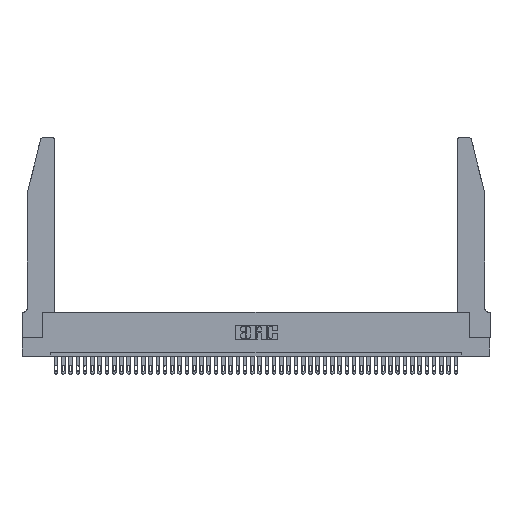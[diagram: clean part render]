
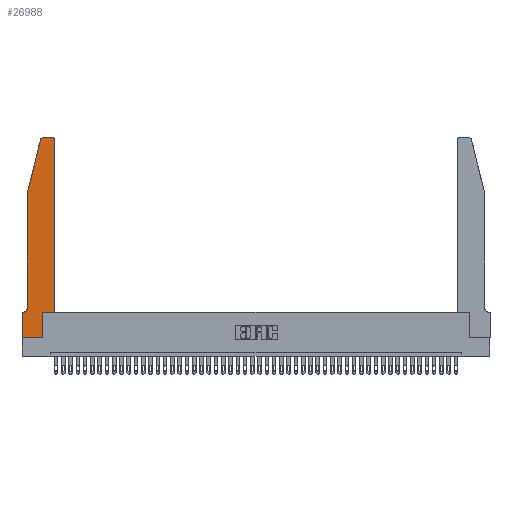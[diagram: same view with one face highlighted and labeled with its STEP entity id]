
A CAD part, top view. The second image highlights one B-rep face of the part: STEP entity #26988.
In plain terms, the highlighted planar face has unit normal (0, 0, 1).
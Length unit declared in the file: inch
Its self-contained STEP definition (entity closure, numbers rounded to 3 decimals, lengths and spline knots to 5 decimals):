
#371 = VERTEX_POINT ( 'NONE', #32483 ) ;
#592 = EDGE_CURVE ( 'NONE', #25665, #30814, #17635, .T. ) ;
#1153 = VERTEX_POINT ( 'NONE', #32497 ) ;
#1251 = CARTESIAN_POINT ( 'NONE',  ( 0.4505, 2.72, 0.37 ) ) ;
#1559 = EDGE_CURVE ( 'NONE', #17417, #25665, #8366, .T. ) ;
#1777 = CARTESIAN_POINT ( 'NONE',  ( 0., 0., 0.37 ) ) ;
#2017 = DIRECTION ( 'NONE',  ( 0., 1., 0. ) ) ;
#2278 = ORIENTED_EDGE ( 'NONE', *, *, #44616, .T. ) ;
#2414 = DIRECTION ( 'NONE',  ( 1., 0., 0. ) ) ;
#2507 = VECTOR ( 'NONE', #15061, 39.37008 ) ;
#2694 = DIRECTION ( 'NONE',  ( 1., 0., 0. ) ) ;
#3032 = DIRECTION ( 'NONE',  ( 0., 0., 1. ) ) ;
#3326 = VERTEX_POINT ( 'NONE', #14627 ) ;
#3653 = AXIS2_PLACEMENT_3D ( 'NONE', #43778, #43934, #2694 ) ;
#4521 = EDGE_CURVE ( 'NONE', #10692, #19245, #15710, .T. ) ;
#5145 = CARTESIAN_POINT ( 'NONE',  ( 0.4505, 0.35, 0.37 ) ) ;
#5306 = VECTOR ( 'NONE', #17128, 39.37008 ) ;
#5864 = CARTESIAN_POINT ( 'NONE',  ( 0.4505, 0.35, 0.37 ) ) ;
#6525 = CARTESIAN_POINT ( 'NONE',  ( 0.0055, 0.35, 0.37 ) ) ;
#7644 = EDGE_CURVE ( 'NONE', #11097, #10396, #30692, .T. ) ;
#8121 = AXIS2_PLACEMENT_3D ( 'NONE', #9512, #3032, #2414 ) ;
#8366 = CIRCLE ( 'NONE', #23593, 0.03 ) ;
#8629 = CARTESIAN_POINT ( 'NONE',  ( 0.284, 2.72, 0.37 ) ) ;
#9006 = EDGE_CURVE ( 'NONE', #23470, #18108, #40958, .T. ) ;
#9471 = VECTOR ( 'NONE', #35552, 39.37008 ) ;
#9512 = CARTESIAN_POINT ( 'NONE',  ( 0., 0.35, 0.37 ) ) ;
#9662 = ORIENTED_EDGE ( 'NONE', *, *, #21331, .T. ) ;
#9673 = PLANE ( 'NONE',  #8121 ) ;
#9804 = DIRECTION ( 'NONE',  ( 1., 0., 0. ) ) ;
#10240 = ORIENTED_EDGE ( 'NONE', *, *, #33646, .T. ) ;
#10396 = VERTEX_POINT ( 'NONE', #38653 ) ;
#10514 = AXIS2_PLACEMENT_3D ( 'NONE', #27894, #14311, #34888 ) ;
#10692 = VERTEX_POINT ( 'NONE', #6525 ) ;
#11011 = LINE ( 'NONE', #29837, #9471 ) ;
#11097 = VERTEX_POINT ( 'NONE', #1777 ) ;
#12189 = ORIENTED_EDGE ( 'NONE', *, *, #9006, .T. ) ;
#13557 = LINE ( 'NONE', #32917, #22737 ) ;
#13656 = VECTOR ( 'NONE', #32850, 39.37008 ) ;
#14247 = ORIENTED_EDGE ( 'NONE', *, *, #39516, .T. ) ;
#14259 = CIRCLE ( 'NONE', #10514, 0.07 ) ;
#14311 = DIRECTION ( 'NONE',  ( 0., 0., -1. ) ) ;
#14452 = CARTESIAN_POINT ( 'NONE',  ( 0.0755, 0.35, 0.37 ) ) ;
#14588 = CARTESIAN_POINT ( 'NONE',  ( 0.25487, 2.72718, 0.37 ) ) ;
#14627 = CARTESIAN_POINT ( 'NONE',  ( 0.4205, 2.75, 0.37 ) ) ;
#14657 = LINE ( 'NONE', #43055, #13656 ) ;
#15061 = DIRECTION ( 'NONE',  ( 1., 0., 0. ) ) ;
#15710 = LINE ( 'NONE', #14452, #38529 ) ;
#16889 = CARTESIAN_POINT ( 'NONE',  ( 0.284, 2.75, 0.37 ) ) ;
#17128 = DIRECTION ( 'NONE',  ( -1., 0., 0. ) ) ;
#17417 = VERTEX_POINT ( 'NONE', #16889 ) ;
#17635 = LINE ( 'NONE', #34402, #20882 ) ;
#18108 = VERTEX_POINT ( 'NONE', #1251 ) ;
#19245 = VERTEX_POINT ( 'NONE', #19876 ) ;
#19876 = CARTESIAN_POINT ( 'NONE',  ( 0., 0.35, 0.37 ) ) ;
#20882 = VECTOR ( 'NONE', #24058, 39.37008 ) ;
#21206 = VECTOR ( 'NONE', #9804, 39.37008 ) ;
#21331 = EDGE_CURVE ( 'NONE', #3326, #17417, #41724, .T. ) ;
#21405 = CARTESIAN_POINT ( 'NONE',  ( 0.0755, 2., 0.37 ) ) ;
#21649 = CIRCLE ( 'NONE', #3653, 0.03 ) ;
#22273 = ORIENTED_EDGE ( 'NONE', *, *, #4521, .T. ) ;
#22362 = VECTOR ( 'NONE', #41183, 39.37008 ) ;
#22737 = VECTOR ( 'NONE', #2017, 39.37008 ) ;
#23470 = VERTEX_POINT ( 'NONE', #5145 ) ;
#23593 = AXIS2_PLACEMENT_3D ( 'NONE', #8629, #32245, #25741 ) ;
#23840 = CARTESIAN_POINT ( 'NONE',  ( 0.4505, 0.35, 0.37 ) ) ;
#24058 = DIRECTION ( 'NONE',  ( -0.239, -0.971, 0. ) ) ;
#24109 = EDGE_CURVE ( 'NONE', #30814, #1153, #11011, .T. ) ;
#24546 = LINE ( 'NONE', #5864, #21206 ) ;
#25665 = VERTEX_POINT ( 'NONE', #14588 ) ;
#25741 = DIRECTION ( 'NONE',  ( 1., 0., 0. ) ) ;
#26988 = ADVANCED_FACE ( 'NONE', ( #29874 ), #9673, .T. ) ;
#27508 = CARTESIAN_POINT ( 'NONE',  ( 0.2605, 2.75, 0.37 ) ) ;
#27894 = CARTESIAN_POINT ( 'NONE',  ( 0.0055, 0.42, 0.37 ) ) ;
#29837 = CARTESIAN_POINT ( 'NONE',  ( 0.0755, 2., 0.37 ) ) ;
#29874 = FACE_OUTER_BOUND ( 'NONE', #32656, .T. ) ;
#30692 = LINE ( 'NONE', #44922, #2507 ) ;
#30759 = ORIENTED_EDGE ( 'NONE', *, *, #1559, .T. ) ;
#30814 = VERTEX_POINT ( 'NONE', #21405 ) ;
#32245 = DIRECTION ( 'NONE',  ( 0., 0., 1. ) ) ;
#32483 = CARTESIAN_POINT ( 'NONE',  ( 0.2865, 0.35, 0.37 ) ) ;
#32497 = CARTESIAN_POINT ( 'NONE',  ( 0.0755, 0.42, 0.37 ) ) ;
#32656 = EDGE_LOOP ( 'NONE', ( #9662, #30759, #41890, #44397, #39322, #22273, #2278, #43233, #14247, #10240, #12189, #44959 ) ) ;
#32797 = EDGE_CURVE ( 'NONE', #1153, #10692, #14259, .T. ) ;
#32850 = DIRECTION ( 'NONE',  ( 0., -1., 0. ) ) ;
#32917 = CARTESIAN_POINT ( 'NONE',  ( 0.2865, 0.35, 0.37 ) ) ;
#33646 = EDGE_CURVE ( 'NONE', #371, #23470, #24546, .T. ) ;
#34402 = CARTESIAN_POINT ( 'NONE',  ( 0.0755, 2., 0.37 ) ) ;
#34888 = DIRECTION ( 'NONE',  ( -1., 0., 0. ) ) ;
#35039 = EDGE_CURVE ( 'NONE', #18108, #3326, #21649, .T. ) ;
#35552 = DIRECTION ( 'NONE',  ( 0., -1., 0. ) ) ;
#38529 = VECTOR ( 'NONE', #38939, 39.37008 ) ;
#38653 = CARTESIAN_POINT ( 'NONE',  ( 0.2865, 0., 0.37 ) ) ;
#38939 = DIRECTION ( 'NONE',  ( -1., 0., 0. ) ) ;
#39322 = ORIENTED_EDGE ( 'NONE', *, *, #32797, .T. ) ;
#39516 = EDGE_CURVE ( 'NONE', #10396, #371, #13557, .T. ) ;
#40958 = LINE ( 'NONE', #23840, #22362 ) ;
#41183 = DIRECTION ( 'NONE',  ( 0., 1., 0. ) ) ;
#41724 = LINE ( 'NONE', #27508, #5306 ) ;
#41890 = ORIENTED_EDGE ( 'NONE', *, *, #592, .T. ) ;
#43055 = CARTESIAN_POINT ( 'NONE',  ( 0., 0., 0.37 ) ) ;
#43233 = ORIENTED_EDGE ( 'NONE', *, *, #7644, .T. ) ;
#43778 = CARTESIAN_POINT ( 'NONE',  ( 0.4205, 2.72, 0.37 ) ) ;
#43934 = DIRECTION ( 'NONE',  ( 0., 0., 1. ) ) ;
#44397 = ORIENTED_EDGE ( 'NONE', *, *, #24109, .T. ) ;
#44616 = EDGE_CURVE ( 'NONE', #19245, #11097, #14657, .T. ) ;
#44922 = CARTESIAN_POINT ( 'NONE',  ( 0., 0., 0.37 ) ) ;
#44959 = ORIENTED_EDGE ( 'NONE', *, *, #35039, .T. ) ;
